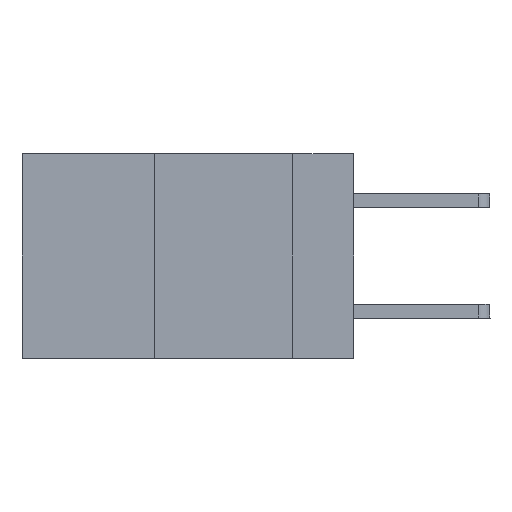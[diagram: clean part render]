
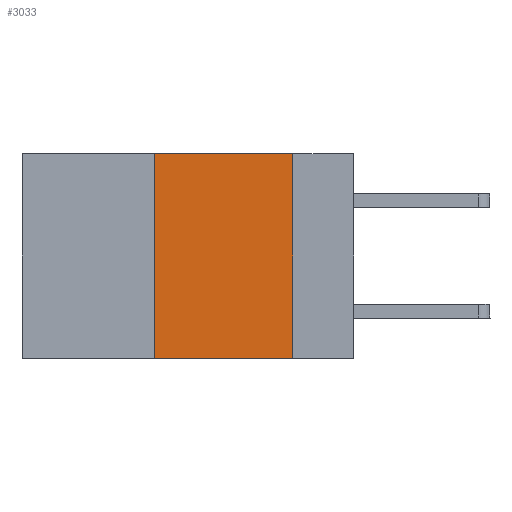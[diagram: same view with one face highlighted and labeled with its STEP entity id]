
A CAD part, left-side view. The second image highlights one B-rep face of the part: STEP entity #3033.
In plain terms, the highlighted planar face has unit normal (-1, 0, 0).
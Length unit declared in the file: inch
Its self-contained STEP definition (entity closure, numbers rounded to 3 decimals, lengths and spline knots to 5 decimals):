
#341 = DIRECTION ( 'NONE',  ( 0., -1., 0. ) ) ;
#837 = PLANE ( 'NONE',  #8185 ) ;
#1084 = CARTESIAN_POINT ( 'NONE',  ( 0., 0.36, 0. ) ) ;
#1385 = EDGE_CURVE ( 'NONE', #11893, #2356, #8037, .T. ) ;
#1414 = VECTOR ( 'NONE', #7842, 39.37008 ) ;
#1666 = LINE ( 'NONE', #10032, #9940 ) ;
#1921 = ORIENTED_EDGE ( 'NONE', *, *, #2828, .F. ) ;
#2356 = VERTEX_POINT ( 'NONE', #5513 ) ;
#2524 = CARTESIAN_POINT ( 'NONE',  ( 0., 0.6, 0. ) ) ;
#2677 = DIRECTION ( 'NONE',  ( 0., 0., -1. ) ) ;
#2828 = EDGE_CURVE ( 'NONE', #6569, #11893, #6799, .T. ) ;
#3033 = ADVANCED_FACE ( 'NONE', ( #7052 ), #837, .F. ) ;
#3422 = DIRECTION ( 'NONE',  ( 0., 0., -1. ) ) ;
#4172 = ORIENTED_EDGE ( 'NONE', *, *, #5853, .T. ) ;
#4807 = EDGE_CURVE ( 'NONE', #2356, #8883, #1666, .T. ) ;
#5113 = CARTESIAN_POINT ( 'NONE',  ( 0., 0.36, 0. ) ) ;
#5513 = CARTESIAN_POINT ( 'NONE',  ( 0., 0.11, 0. ) ) ;
#5853 = EDGE_CURVE ( 'NONE', #6569, #8883, #11197, .T. ) ;
#6140 = CARTESIAN_POINT ( 'NONE',  ( 0., 0.6, 0. ) ) ;
#6569 = VERTEX_POINT ( 'NONE', #11602 ) ;
#6799 = LINE ( 'NONE', #5113, #1414 ) ;
#7052 = FACE_OUTER_BOUND ( 'NONE', #8055, .T. ) ;
#7407 = CARTESIAN_POINT ( 'NONE',  ( 0., 0.6, -0.37 ) ) ;
#7842 = DIRECTION ( 'NONE',  ( 0., 0., 1. ) ) ;
#8037 = LINE ( 'NONE', #2524, #8903 ) ;
#8055 = EDGE_LOOP ( 'NONE', ( #8923, #11701, #1921, #4172 ) ) ;
#8185 = AXIS2_PLACEMENT_3D ( 'NONE', #6140, #8944, #3422 ) ;
#8883 = VERTEX_POINT ( 'NONE', #9237 ) ;
#8903 = VECTOR ( 'NONE', #9939, 39.37008 ) ;
#8923 = ORIENTED_EDGE ( 'NONE', *, *, #4807, .F. ) ;
#8944 = DIRECTION ( 'NONE',  ( 1., 0., 0. ) ) ;
#9237 = CARTESIAN_POINT ( 'NONE',  ( 0., 0.11, -0.37 ) ) ;
#9939 = DIRECTION ( 'NONE',  ( 0., -1., 0. ) ) ;
#9940 = VECTOR ( 'NONE', #2677, 39.37008 ) ;
#10032 = CARTESIAN_POINT ( 'NONE',  ( 0., 0.11, 0. ) ) ;
#11197 = LINE ( 'NONE', #7407, #11942 ) ;
#11602 = CARTESIAN_POINT ( 'NONE',  ( 0., 0.36, -0.37 ) ) ;
#11701 = ORIENTED_EDGE ( 'NONE', *, *, #1385, .F. ) ;
#11893 = VERTEX_POINT ( 'NONE', #1084 ) ;
#11942 = VECTOR ( 'NONE', #341, 39.37008 ) ;
